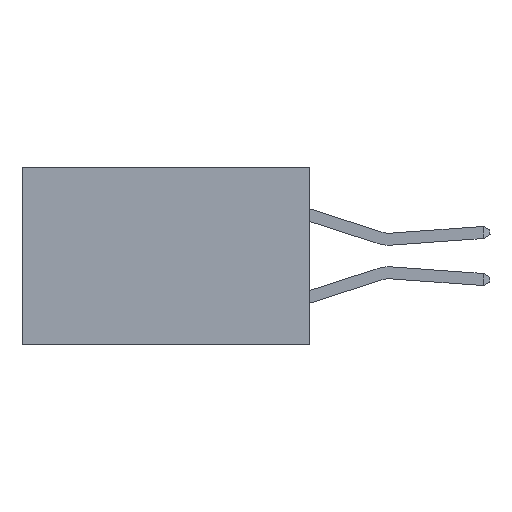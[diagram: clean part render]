
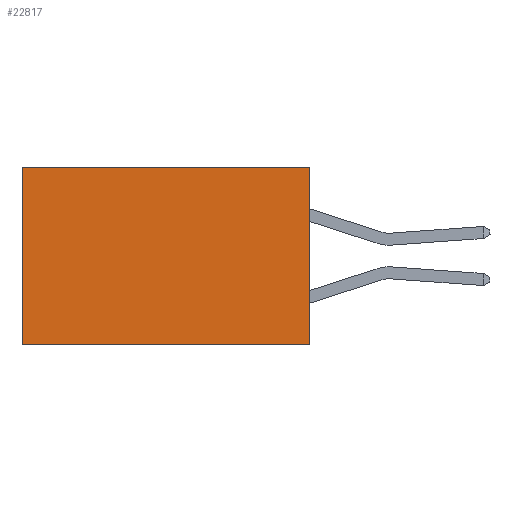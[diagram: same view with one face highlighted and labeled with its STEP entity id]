
A CAD part, left-side view. The second image highlights one B-rep face of the part: STEP entity #22817.
In plain terms, the highlighted planar face has unit normal (-1, 0, 0).
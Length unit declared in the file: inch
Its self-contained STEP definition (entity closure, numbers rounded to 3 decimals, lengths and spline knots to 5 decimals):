
#761 = ORIENTED_EDGE ( 'NONE', *, *, #19634, .T. ) ;
#2200 = DIRECTION ( 'NONE',  ( 1., 0., 0. ) ) ;
#2513 = LINE ( 'NONE', #17455, #10049 ) ;
#2699 = CARTESIAN_POINT ( 'NONE',  ( 0.2615, 0., -0.37 ) ) ;
#2731 = VERTEX_POINT ( 'NONE', #20456 ) ;
#4517 = VERTEX_POINT ( 'NONE', #13061 ) ;
#4523 = DIRECTION ( 'NONE',  ( 0., 0., -1. ) ) ;
#5687 = EDGE_CURVE ( 'NONE', #12580, #2731, #25861, .T. ) ;
#6015 = VERTEX_POINT ( 'NONE', #9132 ) ;
#7678 = DIRECTION ( 'NONE',  ( 0., 0., -1. ) ) ;
#7704 = EDGE_CURVE ( 'NONE', #4517, #12580, #2513, .T. ) ;
#9118 = ORIENTED_EDGE ( 'NONE', *, *, #12803, .T. ) ;
#9132 = CARTESIAN_POINT ( 'NONE',  ( 0.2615, 0.6, 0. ) ) ;
#10049 = VECTOR ( 'NONE', #26076, 39.37008 ) ;
#10256 = EDGE_LOOP ( 'NONE', ( #9118, #14471, #12533, #761 ) ) ;
#10398 = VECTOR ( 'NONE', #12956, 39.37008 ) ;
#11028 = DIRECTION ( 'NONE',  ( 0., 1., 0. ) ) ;
#11977 = CARTESIAN_POINT ( 'NONE',  ( 0.2615, 0.6, -0.37 ) ) ;
#12533 = ORIENTED_EDGE ( 'NONE', *, *, #7704, .F. ) ;
#12580 = VERTEX_POINT ( 'NONE', #2699 ) ;
#12803 = EDGE_CURVE ( 'NONE', #6015, #2731, #26692, .T. ) ;
#12861 = VECTOR ( 'NONE', #11028, 39.37008 ) ;
#12956 = DIRECTION ( 'NONE',  ( 0., 1., 0. ) ) ;
#13061 = CARTESIAN_POINT ( 'NONE',  ( 0.2615, 0., 0. ) ) ;
#14471 = ORIENTED_EDGE ( 'NONE', *, *, #5687, .F. ) ;
#15165 = LINE ( 'NONE', #23654, #12861 ) ;
#16984 = PLANE ( 'NONE',  #18313 ) ;
#17387 = CARTESIAN_POINT ( 'NONE',  ( 0.2615, 0., -0.37 ) ) ;
#17455 = CARTESIAN_POINT ( 'NONE',  ( 0.2615, 0., -0.37 ) ) ;
#18313 = AXIS2_PLACEMENT_3D ( 'NONE', #23539, #2200, #4523 ) ;
#19634 = EDGE_CURVE ( 'NONE', #4517, #6015, #15165, .T. ) ;
#20456 = CARTESIAN_POINT ( 'NONE',  ( 0.2615, 0.6, -0.37 ) ) ;
#20794 = VECTOR ( 'NONE', #7678, 39.37008 ) ;
#21177 = FACE_OUTER_BOUND ( 'NONE', #10256, .T. ) ;
#22817 = ADVANCED_FACE ( 'NONE', ( #21177 ), #16984, .F. ) ;
#23539 = CARTESIAN_POINT ( 'NONE',  ( 0.2615, 0., -0.37 ) ) ;
#23654 = CARTESIAN_POINT ( 'NONE',  ( 0.2615, 0., 0. ) ) ;
#25861 = LINE ( 'NONE', #17387, #10398 ) ;
#26076 = DIRECTION ( 'NONE',  ( 0., 0., -1. ) ) ;
#26692 = LINE ( 'NONE', #11977, #20794 ) ;
